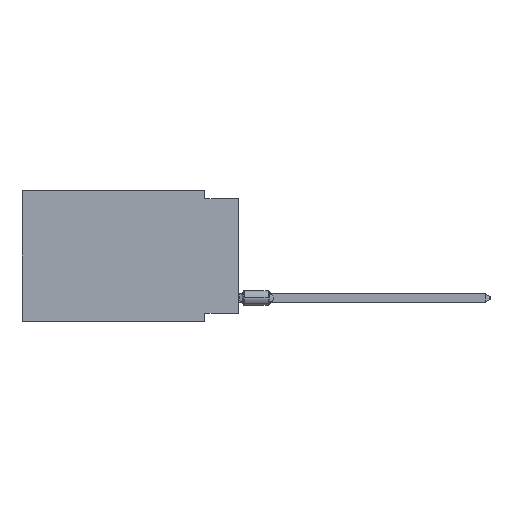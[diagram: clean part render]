
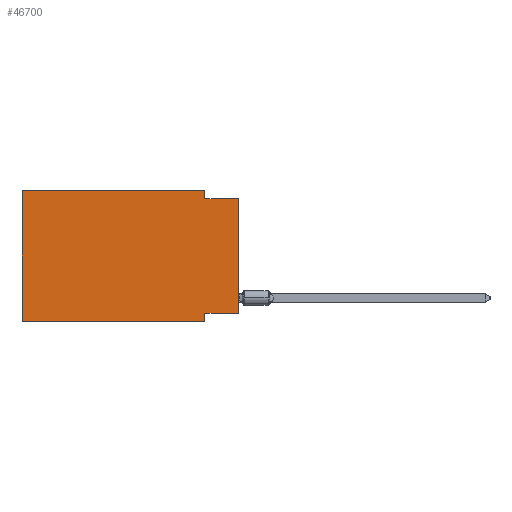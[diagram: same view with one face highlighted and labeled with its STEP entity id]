
A CAD part, left-side view. The second image highlights one B-rep face of the part: STEP entity #46700.
In plain terms, the highlighted planar face has unit normal (-1, 0, 0).
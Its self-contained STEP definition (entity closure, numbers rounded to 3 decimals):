
#486 = LINE ( 'NONE', #25092, #32879 ) ;
#1017 = DIRECTION ( 'NONE',  ( 1., 0., 0. ) ) ;
#2226 = CARTESIAN_POINT ( 'NONE',  ( 0., 16.383, 0. ) ) ;
#3852 = CARTESIAN_POINT ( 'NONE',  ( 0., 2.54, 0. ) ) ;
#4193 = EDGE_CURVE ( 'NONE', #33286, #39170, #51090, .T. ) ;
#4859 = DIRECTION ( 'NONE',  ( 0., -1., 0. ) ) ;
#6718 = CARTESIAN_POINT ( 'NONE',  ( 0., 16.383, 0. ) ) ;
#7019 = EDGE_CURVE ( 'NONE', #33286, #19721, #52854, .T. ) ;
#7323 = ORIENTED_EDGE ( 'NONE', *, *, #40582, .F. ) ;
#8138 = CARTESIAN_POINT ( 'NONE',  ( 0., 0., -0.635 ) ) ;
#8485 = VECTOR ( 'NONE', #43947, 1000. ) ;
#9258 = VERTEX_POINT ( 'NONE', #25011 ) ;
#9573 = VECTOR ( 'NONE', #29415, 1000. ) ;
#10644 = ORIENTED_EDGE ( 'NONE', *, *, #47354, .T. ) ;
#11883 = VECTOR ( 'NONE', #46004, 1000. ) ;
#16319 = ORIENTED_EDGE ( 'NONE', *, *, #7019, .F. ) ;
#16370 = DIRECTION ( 'NONE',  ( 0., 0., -1. ) ) ;
#17422 = CARTESIAN_POINT ( 'NONE',  ( 0., 16.383, 0. ) ) ;
#17436 = CARTESIAN_POINT ( 'NONE',  ( 0., 16.383, 0. ) ) ;
#17647 = CARTESIAN_POINT ( 'NONE',  ( 0., 0., 0. ) ) ;
#18258 = VECTOR ( 'NONE', #34269, 1000. ) ;
#19112 = EDGE_LOOP ( 'NONE', ( #45542, #41881, #27016, #51812, #45852, #10644, #7323, #16319 ) ) ;
#19721 = VERTEX_POINT ( 'NONE', #34555 ) ;
#19789 = CARTESIAN_POINT ( 'NONE',  ( 0., 2.54, 0. ) ) ;
#21258 = DIRECTION ( 'NONE',  ( 0., 0., -1. ) ) ;
#22979 = CARTESIAN_POINT ( 'NONE',  ( 0., 0., -9.271 ) ) ;
#23083 = EDGE_CURVE ( 'NONE', #25648, #39170, #49803, .T. ) ;
#23562 = AXIS2_PLACEMENT_3D ( 'NONE', #17436, #1017, #21258 ) ;
#23769 = VECTOR ( 'NONE', #27611, 1000. ) ;
#24167 = DIRECTION ( 'NONE',  ( 0., 0., -1. ) ) ;
#25011 = CARTESIAN_POINT ( 'NONE',  ( 0., 16.383, -9.906 ) ) ;
#25090 = EDGE_CURVE ( 'NONE', #9258, #53849, #39605, .T. ) ;
#25092 = CARTESIAN_POINT ( 'NONE',  ( 0., 2.54, -9.906 ) ) ;
#25317 = LINE ( 'NONE', #29163, #9573 ) ;
#25648 = VERTEX_POINT ( 'NONE', #46668 ) ;
#27016 = ORIENTED_EDGE ( 'NONE', *, *, #41828, .F. ) ;
#27387 = VECTOR ( 'NONE', #4859, 1000. ) ;
#27611 = DIRECTION ( 'NONE',  ( 0., 1., 0. ) ) ;
#27862 = VECTOR ( 'NONE', #24167, 1000. ) ;
#29163 = CARTESIAN_POINT ( 'NONE',  ( 0., 16.383, -9.906 ) ) ;
#29415 = DIRECTION ( 'NONE',  ( 0., -1., 0. ) ) ;
#32879 = VECTOR ( 'NONE', #16370, 1000. ) ;
#33286 = VERTEX_POINT ( 'NONE', #43399 ) ;
#34269 = DIRECTION ( 'NONE',  ( 0., 0., 1. ) ) ;
#34555 = CARTESIAN_POINT ( 'NONE',  ( 0., 2.54, -9.271 ) ) ;
#39170 = VERTEX_POINT ( 'NONE', #43093 ) ;
#39605 = LINE ( 'NONE', #2226, #8485 ) ;
#40582 = EDGE_CURVE ( 'NONE', #19721, #45699, #486, .T. ) ;
#40958 = VERTEX_POINT ( 'NONE', #3852 ) ;
#41828 = EDGE_CURVE ( 'NONE', #40958, #25648, #53232, .T. ) ;
#41881 = ORIENTED_EDGE ( 'NONE', *, *, #23083, .F. ) ;
#43093 = CARTESIAN_POINT ( 'NONE',  ( 0., 0., -0.635 ) ) ;
#43399 = CARTESIAN_POINT ( 'NONE',  ( 0., 0., -9.271 ) ) ;
#43947 = DIRECTION ( 'NONE',  ( 0., 0., 1. ) ) ;
#45471 = EDGE_CURVE ( 'NONE', #53849, #40958, #50331, .T. ) ;
#45542 = ORIENTED_EDGE ( 'NONE', *, *, #4193, .T. ) ;
#45699 = VERTEX_POINT ( 'NONE', #49472 ) ;
#45852 = ORIENTED_EDGE ( 'NONE', *, *, #25090, .F. ) ;
#46004 = DIRECTION ( 'NONE',  ( 0., -1., 0. ) ) ;
#46668 = CARTESIAN_POINT ( 'NONE',  ( 0., 2.54, -0.635 ) ) ;
#46700 = ADVANCED_FACE ( 'NONE', ( #50615 ), #50890, .F. ) ;
#47354 = EDGE_CURVE ( 'NONE', #9258, #45699, #25317, .T. ) ;
#49472 = CARTESIAN_POINT ( 'NONE',  ( 0., 2.54, -9.906 ) ) ;
#49803 = LINE ( 'NONE', #8138, #27387 ) ;
#50331 = LINE ( 'NONE', #17422, #11883 ) ;
#50615 = FACE_OUTER_BOUND ( 'NONE', #19112, .T. ) ;
#50890 = PLANE ( 'NONE',  #23562 ) ;
#51090 = LINE ( 'NONE', #17647, #18258 ) ;
#51812 = ORIENTED_EDGE ( 'NONE', *, *, #45471, .F. ) ;
#52854 = LINE ( 'NONE', #22979, #23769 ) ;
#53232 = LINE ( 'NONE', #19789, #27862 ) ;
#53849 = VERTEX_POINT ( 'NONE', #6718 ) ;
